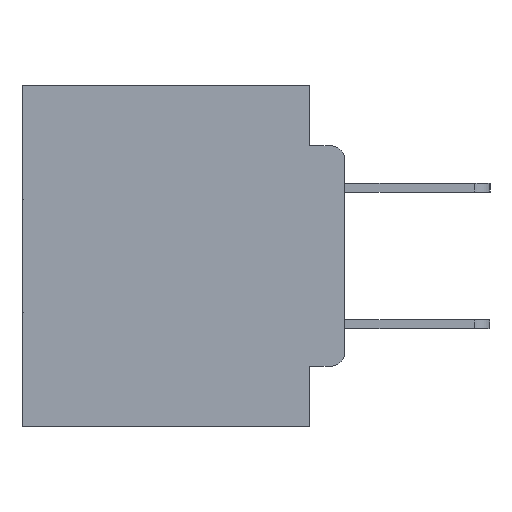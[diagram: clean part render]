
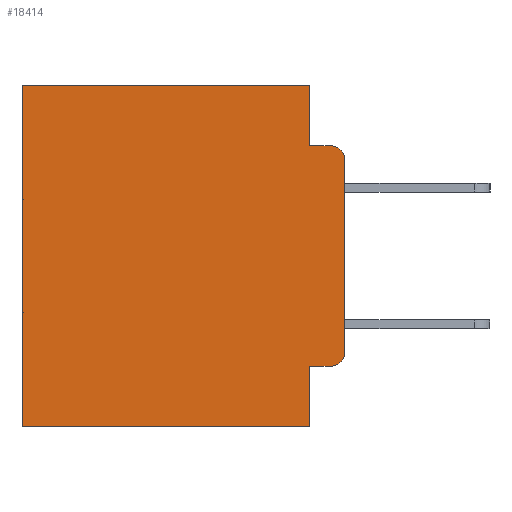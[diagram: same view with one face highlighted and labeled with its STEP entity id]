
A CAD part, left-side view. The second image highlights one B-rep face of the part: STEP entity #18414.
In plain terms, the highlighted planar face has unit normal (-1, 0, 0).
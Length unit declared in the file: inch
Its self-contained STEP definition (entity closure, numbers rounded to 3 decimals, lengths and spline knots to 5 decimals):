
#183 = VECTOR ( 'NONE', #23618, 39.37008 ) ;
#246 = CARTESIAN_POINT ( 'NONE',  ( 0.298, 0., -0.3915 ) ) ;
#458 = LINE ( 'NONE', #27522, #25453 ) ;
#537 = CARTESIAN_POINT ( 'NONE',  ( 0.298, 0.051, -0.0885 ) ) ;
#827 = CARTESIAN_POINT ( 'NONE',  ( 0.298, 0.02, -0.4115 ) ) ;
#969 = EDGE_CURVE ( 'NONE', #15303, #986, #458, .T. ) ;
#986 = VERTEX_POINT ( 'NONE', #246 ) ;
#1284 = LINE ( 'NONE', #9942, #7027 ) ;
#1394 = EDGE_CURVE ( 'NONE', #24906, #18722, #20835, .T. ) ;
#1864 = DIRECTION ( 'NONE',  ( 0., 0., -1. ) ) ;
#2048 = FACE_OUTER_BOUND ( 'NONE', #21777, .T. ) ;
#2418 = EDGE_CURVE ( 'NONE', #16706, #9470, #24672, .T. ) ;
#2541 = AXIS2_PLACEMENT_3D ( 'NONE', #7294, #23540, #9692 ) ;
#3593 = ORIENTED_EDGE ( 'NONE', *, *, #26083, .F. ) ;
#4129 = CARTESIAN_POINT ( 'NONE',  ( 0.298, 0., -0.1085 ) ) ;
#4702 = CARTESIAN_POINT ( 'NONE',  ( 0.298, 0., 0. ) ) ;
#5384 = AXIS2_PLACEMENT_3D ( 'NONE', #29685, #16167, #1864 ) ;
#6175 = CARTESIAN_POINT ( 'NONE',  ( 0.298, 0.473, -0.5 ) ) ;
#6246 = DIRECTION ( 'NONE',  ( 0., -1., 0. ) ) ;
#6628 = DIRECTION ( 'NONE',  ( 0., 0., -1. ) ) ;
#6653 = DIRECTION ( 'NONE',  ( 0., 0., -1. ) ) ;
#6914 = PLANE ( 'NONE',  #12645 ) ;
#7027 = VECTOR ( 'NONE', #28231, 39.37008 ) ;
#7294 = CARTESIAN_POINT ( 'NONE',  ( 0.298, 0.02, -0.3915 ) ) ;
#7478 = LINE ( 'NONE', #21330, #183 ) ;
#8280 = VERTEX_POINT ( 'NONE', #30093 ) ;
#8485 = VECTOR ( 'NONE', #26551, 39.37008 ) ;
#9244 = ORIENTED_EDGE ( 'NONE', *, *, #27536, .F. ) ;
#9308 = DIRECTION ( 'NONE',  ( 1., 0., 0. ) ) ;
#9470 = VERTEX_POINT ( 'NONE', #27331 ) ;
#9692 = DIRECTION ( 'NONE',  ( 0., 0., -1. ) ) ;
#9942 = CARTESIAN_POINT ( 'NONE',  ( 0.298, 0.051, -0.4115 ) ) ;
#10805 = VERTEX_POINT ( 'NONE', #537 ) ;
#11591 = VECTOR ( 'NONE', #6246, 39.37008 ) ;
#11831 = ORIENTED_EDGE ( 'NONE', *, *, #28088, .T. ) ;
#12268 = EDGE_CURVE ( 'NONE', #15303, #8280, #18752, .T. ) ;
#12645 = AXIS2_PLACEMENT_3D ( 'NONE', #23182, #9308, #25416 ) ;
#13669 = CARTESIAN_POINT ( 'NONE',  ( 0.298, 0.051, 0. ) ) ;
#15058 = ORIENTED_EDGE ( 'NONE', *, *, #2418, .F. ) ;
#15303 = VERTEX_POINT ( 'NONE', #4129 ) ;
#15351 = CARTESIAN_POINT ( 'NONE',  ( 0.298, 0.051, 0. ) ) ;
#15477 = EDGE_CURVE ( 'NONE', #19911, #986, #24918, .T. ) ;
#15488 = ORIENTED_EDGE ( 'NONE', *, *, #19445, .F. ) ;
#15798 = ORIENTED_EDGE ( 'NONE', *, *, #15477, .T. ) ;
#16167 = DIRECTION ( 'NONE',  ( -1., 0., 0. ) ) ;
#16383 = CARTESIAN_POINT ( 'NONE',  ( 0.298, 0.051, -0.4115 ) ) ;
#16406 = VERTEX_POINT ( 'NONE', #15351 ) ;
#16706 = VERTEX_POINT ( 'NONE', #16383 ) ;
#16916 = ORIENTED_EDGE ( 'NONE', *, *, #18455, .T. ) ;
#18414 = ADVANCED_FACE ( 'NONE', ( #2048 ), #6914, .F. ) ;
#18455 = EDGE_CURVE ( 'NONE', #16706, #19911, #1284, .T. ) ;
#18564 = ORIENTED_EDGE ( 'NONE', *, *, #969, .F. ) ;
#18722 = VERTEX_POINT ( 'NONE', #6175 ) ;
#18752 = CIRCLE ( 'NONE', #5384, 0.02 ) ;
#19445 = EDGE_CURVE ( 'NONE', #16406, #10805, #23334, .T. ) ;
#19911 = VERTEX_POINT ( 'NONE', #827 ) ;
#20835 = LINE ( 'NONE', #22147, #8485 ) ;
#20913 = VECTOR ( 'NONE', #27852, 39.37008 ) ;
#21330 = CARTESIAN_POINT ( 'NONE',  ( 0.298, 0., -0.5 ) ) ;
#21777 = EDGE_LOOP ( 'NONE', ( #18564, #24940, #3593, #15488, #11831, #23013, #9244, #15058, #16916, #15798 ) ) ;
#22147 = CARTESIAN_POINT ( 'NONE',  ( 0.298, 0.473, 0. ) ) ;
#22540 = CARTESIAN_POINT ( 'NONE',  ( 0.298, 0.051, -0.0885 ) ) ;
#22623 = VECTOR ( 'NONE', #6653, 39.37008 ) ;
#23013 = ORIENTED_EDGE ( 'NONE', *, *, #1394, .T. ) ;
#23182 = CARTESIAN_POINT ( 'NONE',  ( 0.298, 0., 0. ) ) ;
#23334 = LINE ( 'NONE', #13669, #22623 ) ;
#23540 = DIRECTION ( 'NONE',  ( -1., 0., 0. ) ) ;
#23618 = DIRECTION ( 'NONE',  ( 0., 1., 0. ) ) ;
#23984 = VECTOR ( 'NONE', #6628, 39.37008 ) ;
#24672 = LINE ( 'NONE', #28890, #23984 ) ;
#24906 = VERTEX_POINT ( 'NONE', #27397 ) ;
#24918 = CIRCLE ( 'NONE', #2541, 0.02 ) ;
#24940 = ORIENTED_EDGE ( 'NONE', *, *, #12268, .T. ) ;
#25416 = DIRECTION ( 'NONE',  ( 0., 0., -1. ) ) ;
#25453 = VECTOR ( 'NONE', #27556, 39.37008 ) ;
#26083 = EDGE_CURVE ( 'NONE', #10805, #8280, #29070, .T. ) ;
#26551 = DIRECTION ( 'NONE',  ( 0., 0., -1. ) ) ;
#26884 = LINE ( 'NONE', #4702, #20913 ) ;
#27331 = CARTESIAN_POINT ( 'NONE',  ( 0.298, 0.051, -0.5 ) ) ;
#27397 = CARTESIAN_POINT ( 'NONE',  ( 0.298, 0.473, 0. ) ) ;
#27522 = CARTESIAN_POINT ( 'NONE',  ( 0.298, 0., 0. ) ) ;
#27536 = EDGE_CURVE ( 'NONE', #9470, #18722, #7478, .T. ) ;
#27556 = DIRECTION ( 'NONE',  ( 0., 0., -1. ) ) ;
#27852 = DIRECTION ( 'NONE',  ( 0., 1., 0. ) ) ;
#28088 = EDGE_CURVE ( 'NONE', #16406, #24906, #26884, .T. ) ;
#28231 = DIRECTION ( 'NONE',  ( 0., -1., 0. ) ) ;
#28890 = CARTESIAN_POINT ( 'NONE',  ( 0.298, 0.051, 0. ) ) ;
#29070 = LINE ( 'NONE', #22540, #11591 ) ;
#29685 = CARTESIAN_POINT ( 'NONE',  ( 0.298, 0.02, -0.1085 ) ) ;
#30093 = CARTESIAN_POINT ( 'NONE',  ( 0.298, 0.02, -0.0885 ) ) ;
